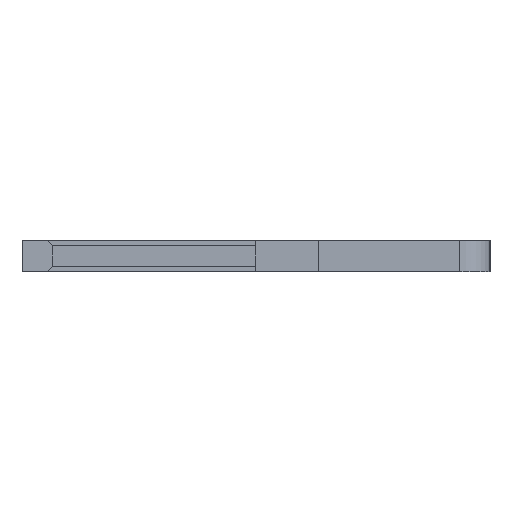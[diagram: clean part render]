
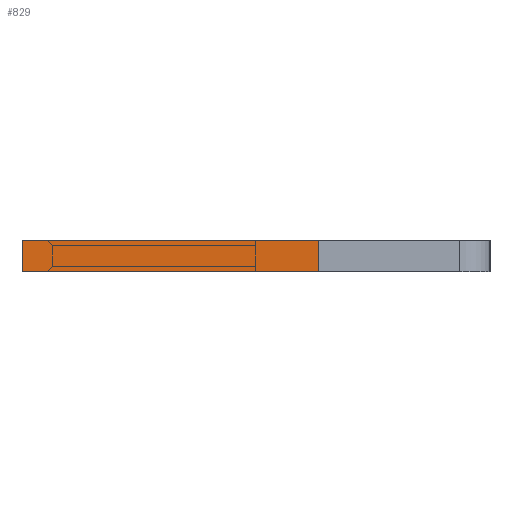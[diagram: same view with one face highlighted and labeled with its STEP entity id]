
A CAD part, left-side view. The second image highlights one B-rep face of the part: STEP entity #829.
In plain terms, the highlighted face is planar.
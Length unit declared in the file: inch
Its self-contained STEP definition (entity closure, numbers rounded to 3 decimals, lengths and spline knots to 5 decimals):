
#14 = LINE ( 'NONE', #470, #286 ) ;
#86 = VERTEX_POINT ( 'NONE', #385 ) ;
#119 = CARTESIAN_POINT ( 'NONE',  ( 0.01, 0.15, -0.04 ) ) ;
#164 = EDGE_CURVE ( 'NONE', #1208, #1759, #538, .T. ) ;
#196 = ORIENTED_EDGE ( 'NONE', *, *, #2171, .T. ) ;
#235 = LINE ( 'NONE', #717, #682 ) ;
#250 = ORIENTED_EDGE ( 'NONE', *, *, #164, .F. ) ;
#286 = VECTOR ( 'NONE', #1229, 39.37008 ) ;
#385 = CARTESIAN_POINT ( 'NONE',  ( -0.01, -0.04, -0.04 ) ) ;
#470 = CARTESIAN_POINT ( 'NONE',  ( -0.01, 0.15, -0.04 ) ) ;
#538 = LINE ( 'NONE', #1178, #599 ) ;
#599 = VECTOR ( 'NONE', #778, 39.37008 ) ;
#635 = DIRECTION ( 'NONE',  ( 0., 0., 1. ) ) ;
#682 = VECTOR ( 'NONE', #1677, 39.37008 ) ;
#684 = FACE_OUTER_BOUND ( 'NONE', #1629, .T. ) ;
#717 = CARTESIAN_POINT ( 'NONE',  ( 0.01, -0.04, -0.04 ) ) ;
#778 = DIRECTION ( 'NONE',  ( 0., 1., 0. ) ) ;
#829 = ADVANCED_FACE ( 'NONE', ( #684 ), #2182, .F. ) ;
#857 = CARTESIAN_POINT ( 'NONE',  ( 0.01, -0.04, -0.04 ) ) ;
#992 = ORIENTED_EDGE ( 'NONE', *, *, #1193, .T. ) ;
#1038 = CARTESIAN_POINT ( 'NONE',  ( 0.01, 0.15, -0.04 ) ) ;
#1171 = VERTEX_POINT ( 'NONE', #1405 ) ;
#1178 = CARTESIAN_POINT ( 'NONE',  ( 0.01, 0.15, -0.04 ) ) ;
#1193 = EDGE_CURVE ( 'NONE', #86, #1171, #14, .T. ) ;
#1208 = VERTEX_POINT ( 'NONE', #857 ) ;
#1229 = DIRECTION ( 'NONE',  ( 0., 1., 0. ) ) ;
#1405 = CARTESIAN_POINT ( 'NONE',  ( -0.01, 0.15, -0.04 ) ) ;
#1514 = AXIS2_PLACEMENT_3D ( 'NONE', #1038, #635, #1604 ) ;
#1604 = DIRECTION ( 'NONE',  ( 1., 0., 0. ) ) ;
#1629 = EDGE_LOOP ( 'NONE', ( #992, #2101, #250, #196 ) ) ;
#1661 = EDGE_CURVE ( 'NONE', #1759, #1171, #1852, .T. ) ;
#1672 = VECTOR ( 'NONE', #2191, 39.37008 ) ;
#1677 = DIRECTION ( 'NONE',  ( -1., 0., 0. ) ) ;
#1759 = VERTEX_POINT ( 'NONE', #119 ) ;
#1852 = LINE ( 'NONE', #2015, #1672 ) ;
#2015 = CARTESIAN_POINT ( 'NONE',  ( 0.01, 0.15, -0.04 ) ) ;
#2101 = ORIENTED_EDGE ( 'NONE', *, *, #1661, .F. ) ;
#2171 = EDGE_CURVE ( 'NONE', #1208, #86, #235, .T. ) ;
#2182 = PLANE ( 'NONE',  #1514 ) ;
#2191 = DIRECTION ( 'NONE',  ( -1., 0., 0. ) ) ;
